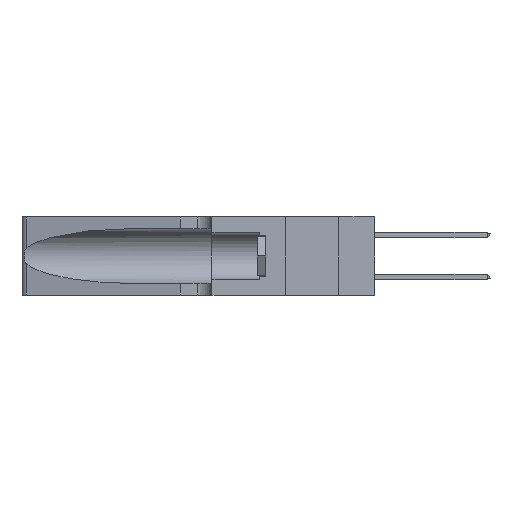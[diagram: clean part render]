
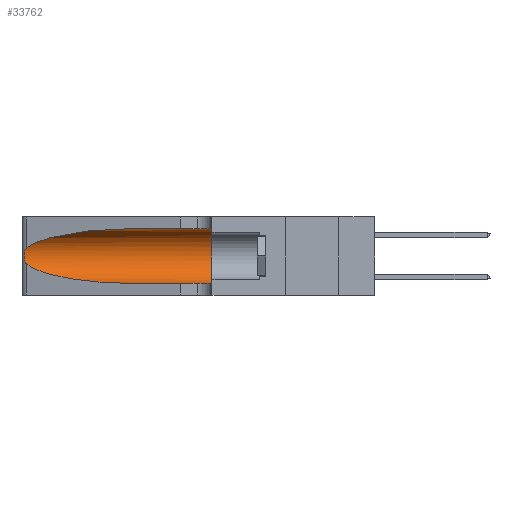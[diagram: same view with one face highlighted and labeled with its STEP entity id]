
A CAD part, left-side view. The second image highlights one B-rep face of the part: STEP entity #33762.
In plain terms, the highlighted cylindrical face has radius 3.308 mm (diameter 6.617 mm), a partial arc.
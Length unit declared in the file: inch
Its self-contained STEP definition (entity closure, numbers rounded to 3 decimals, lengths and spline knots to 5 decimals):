
#2079 = CARTESIAN_POINT ( 'NONE',  ( 0.26075, 1.23896, 0.178 ) ) ;
#2622 = DIRECTION ( 'NONE',  ( 0., -1., 0. ) ) ;
#4857 = ORIENTED_EDGE ( 'NONE', *, *, #38250, .F. ) ;
#5840 = CARTESIAN_POINT ( 'NONE',  ( 0.25856, 1.23593, 0.16098 ) ) ;
#6039 = CARTESIAN_POINT ( 'NONE',  ( 0.1305, 0.35, 0.185 ) ) ;
#7060 =( BOUNDED_CURVE ( )  B_SPLINE_CURVE ( 3, ( #40296, #29485, #7307, #33135 ),
 .UNSPECIFIED., .F., .F. ) 
 B_SPLINE_CURVE_WITH_KNOTS ( ( 4, 4 ),
 ( 1.5708, 2.84003 ),
 .UNSPECIFIED. ) 
 CURVE ( )  GEOMETRIC_REPRESENTATION_ITEM ( )  RATIONAL_B_SPLINE_CURVE ( ( 1., 0.87, 0.87, 1. ) ) 
 REPRESENTATION_ITEM ( '' )  );
#7307 = CARTESIAN_POINT ( 'NONE',  ( 0.2373, 1.15595, 0.28018 ) ) ;
#8927 = LINE ( 'NONE', #21225, #45632 ) ;
#9602 = CARTESIAN_POINT ( 'NONE',  ( 0.25639, 1.23186, 0.15144 ) ) ;
#9631 = CARTESIAN_POINT ( 'NONE',  ( 0.2373, 1.15595, 0.08982 ) ) ;
#9799 = DIRECTION ( 'NONE',  ( 0., 0., 1. ) ) ;
#9889 = AXIS2_PLACEMENT_3D ( 'NONE', #21879, #25569, #43693 ) ;
#10669 = B_SPLINE_CURVE_WITH_KNOTS ( 'NONE', 3,
 ( #16930, #24234, #13179, #42521, #20666, #46142, #24385, #2079, #28043, #5840, #31700, #9602, #35358, #13350 ),
 .UNSPECIFIED., .F., .F.,
 ( 4, 2, 2, 2, 2, 2, 4 ),
 ( 0., 0.00027, 0.00053, 0.00107, 0.0016, 0.00187, 0.00214 ),
 .UNSPECIFIED. ) ;
#12009 = EDGE_CURVE ( 'NONE', #45337, #20699, #10669, .T. ) ;
#13179 = CARTESIAN_POINT ( 'NONE',  ( 0.25639, 1.23184, 0.21858 ) ) ;
#13350 = CARTESIAN_POINT ( 'NONE',  ( 0.25487, 1.22718, 0.14631 ) ) ;
#13524 = CARTESIAN_POINT ( 'NONE',  ( 0.1305, 1.61858, 0.05475 ) ) ;
#13565 = EDGE_CURVE ( 'NONE', #28789, #22939, #24991, .T. ) ;
#16118 = ORIENTED_EDGE ( 'NONE', *, *, #40757, .T. ) ;
#16456 = ORIENTED_EDGE ( 'NONE', *, *, #12009, .T. ) ;
#16930 = CARTESIAN_POINT ( 'NONE',  ( 0.25487, 1.22718, 0.22369 ) ) ;
#19103 = FACE_OUTER_BOUND ( 'NONE', #28880, .T. ) ;
#20320 = VERTEX_POINT ( 'NONE', #33544 ) ;
#20666 = CARTESIAN_POINT ( 'NONE',  ( 0.25854, 1.2359, 0.20912 ) ) ;
#20699 = VERTEX_POINT ( 'NONE', #39391 ) ;
#20859 = CARTESIAN_POINT ( 'NONE',  ( 0.1305, 0.72297, 0.05475 ) ) ;
#21225 = CARTESIAN_POINT ( 'NONE',  ( 0.1305, 1.61858, 0.31525 ) ) ;
#21879 = CARTESIAN_POINT ( 'NONE',  ( 0.1305, 1.61858, 0.185 ) ) ;
#21988 = ORIENTED_EDGE ( 'NONE', *, *, #36002, .T. ) ;
#22939 = VERTEX_POINT ( 'NONE', #25601 ) ;
#24234 = CARTESIAN_POINT ( 'NONE',  ( 0.25555, 1.22994, 0.2215 ) ) ;
#24385 = CARTESIAN_POINT ( 'NONE',  ( 0.26075, 1.23896, 0.19203 ) ) ;
#24991 = CIRCLE ( 'NONE', #35074, 0.13025 ) ;
#25569 = DIRECTION ( 'NONE',  ( 0., -1., 0. ) ) ;
#25601 = CARTESIAN_POINT ( 'NONE',  ( 0.1305, 0.35, 0.05475 ) ) ;
#26286 = CARTESIAN_POINT ( 'NONE',  ( 0.25487, 1.22718, 0.22369 ) ) ;
#28043 = CARTESIAN_POINT ( 'NONE',  ( 0.26017, 1.23833, 0.17102 ) ) ;
#28684 = EDGE_CURVE ( 'NONE', #20320, #22939, #28804, .T. ) ;
#28789 = VERTEX_POINT ( 'NONE', #35439 ) ;
#28804 = LINE ( 'NONE', #13524, #37353 ) ;
#28880 = EDGE_LOOP ( 'NONE', ( #21988, #16456, #16118, #36657, #32551, #4857 ) ) ;
#29485 = CARTESIAN_POINT ( 'NONE',  ( 0.18966, 0.96281, 0.31525 ) ) ;
#31158 = VERTEX_POINT ( 'NONE', #33329 ) ;
#31700 = CARTESIAN_POINT ( 'NONE',  ( 0.25789, 1.23486, 0.15765 ) ) ;
#31900 = DIRECTION ( 'NONE',  ( 0., 1., 0. ) ) ;
#32551 = ORIENTED_EDGE ( 'NONE', *, *, #13565, .F. ) ;
#33135 = CARTESIAN_POINT ( 'NONE',  ( 0.25487, 1.22718, 0.22369 ) ) ;
#33329 = CARTESIAN_POINT ( 'NONE',  ( 0.1305, 0.72297, 0.31525 ) ) ;
#33544 = CARTESIAN_POINT ( 'NONE',  ( 0.1305, 0.72297, 0.05475 ) ) ;
#33762 = ADVANCED_FACE ( 'NONE', ( #19103 ), #37403, .F. ) ;
#35074 = AXIS2_PLACEMENT_3D ( 'NONE', #6039, #31900, #9799 ) ;
#35358 = CARTESIAN_POINT ( 'NONE',  ( 0.25555, 1.22993, 0.14849 ) ) ;
#35382 = CARTESIAN_POINT ( 'NONE',  ( 0.25487, 1.22718, 0.14631 ) ) ;
#35439 = CARTESIAN_POINT ( 'NONE',  ( 0.1305, 0.35, 0.31525 ) ) ;
#36002 = EDGE_CURVE ( 'NONE', #31158, #45337, #7060, .T. ) ;
#36657 = ORIENTED_EDGE ( 'NONE', *, *, #28684, .T. ) ;
#37353 = VECTOR ( 'NONE', #42845, 39.37008 ) ;
#37403 = CYLINDRICAL_SURFACE ( 'NONE', #9889, 0.13025 ) ;
#38250 = EDGE_CURVE ( 'NONE', #31158, #28789, #8927, .T. ) ;
#39391 = CARTESIAN_POINT ( 'NONE',  ( 0.25487, 1.22718, 0.14631 ) ) ;
#40296 = CARTESIAN_POINT ( 'NONE',  ( 0.1305, 0.72297, 0.31525 ) ) ;
#40757 = EDGE_CURVE ( 'NONE', #20699, #20320, #46200, .T. ) ;
#42521 = CARTESIAN_POINT ( 'NONE',  ( 0.25787, 1.23484, 0.2124 ) ) ;
#42699 = CARTESIAN_POINT ( 'NONE',  ( 0.18966, 0.96281, 0.05475 ) ) ;
#42845 = DIRECTION ( 'NONE',  ( 0., -1., 0. ) ) ;
#43693 = DIRECTION ( 'NONE',  ( 0., 0., -1. ) ) ;
#45337 = VERTEX_POINT ( 'NONE', #26286 ) ;
#45632 = VECTOR ( 'NONE', #2622, 39.37008 ) ;
#46142 = CARTESIAN_POINT ( 'NONE',  ( 0.26018, 1.23835, 0.19895 ) ) ;
#46200 =( BOUNDED_CURVE ( )  B_SPLINE_CURVE ( 3, ( #35382, #9631, #42699, #20859 ),
 .UNSPECIFIED., .F., .F. ) 
 B_SPLINE_CURVE_WITH_KNOTS ( ( 4, 4 ),
 ( 3.44316, 4.71239 ),
 .UNSPECIFIED. ) 
 CURVE ( )  GEOMETRIC_REPRESENTATION_ITEM ( )  RATIONAL_B_SPLINE_CURVE ( ( 1., 0.87, 0.87, 1. ) ) 
 REPRESENTATION_ITEM ( '' )  );
